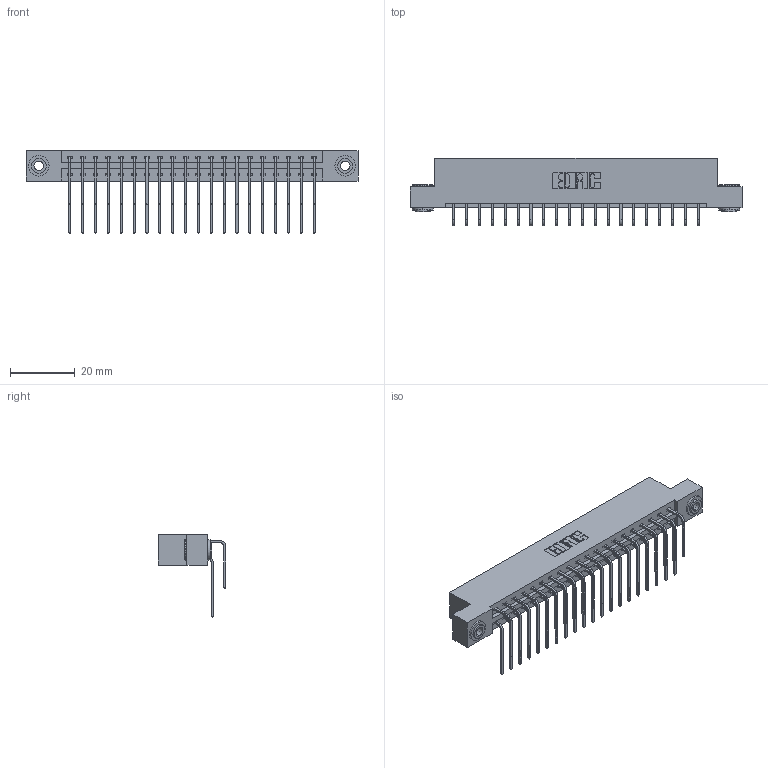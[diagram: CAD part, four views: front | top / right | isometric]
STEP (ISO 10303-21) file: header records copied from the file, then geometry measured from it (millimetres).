
FILE_DESCRIPTION (( 'STEP AP203' ), '1' );
FILE_NAME ('337-040-559-203.STEP', '2018-08-08T20:46:17', ( '' ), ( '' ), 'SwSTEP 2.0', 'SolidWorks 2016', '' );
FILE_SCHEMA (( 'CONFIG_CONTROL_DESIGN' ));
Length unit declared in the file: inch
Products named in the file (5): 337 Part_Flush Mounting Lugs - 0.156 Dia-TH; 345-292-001_558 559 Tail - 1; 345-292-001_559 Tail - 2; 345-250-002_345-250-002-102; 337-040-559-203
Assembly tree (43 placements, depth 2):
  337-040-559-203
    337 Part_Flush Mounting Lugs - 0.156 Dia-TH
    345-292-001_558 559 Tail - 1  x20
    345-292-001_559 Tail - 2  x20
    345-250-002_345-250-002-102  x2
Bounding box: 102.26 x 20.9 x 25.53 mm (x, y, z)
Volume: 10734.3 mm3; surface area: 13304.5 mm2
Topology: 43 solids, 43 shells, 2392 faces, 7067 edges, 4654 vertices
Faces by surface type: plane 1680, cylinder 704, cone 8
Entity records: 20786 total; most frequent: CARTESIAN_POINT 3540, ORIENTED_EDGE 3418, DIRECTION 3067, EDGE_CURVE 1709, VECTOR 1517, LINE 1517, VERTEX_POINT 1134, AXIS2_PLACEMENT_3D 775
